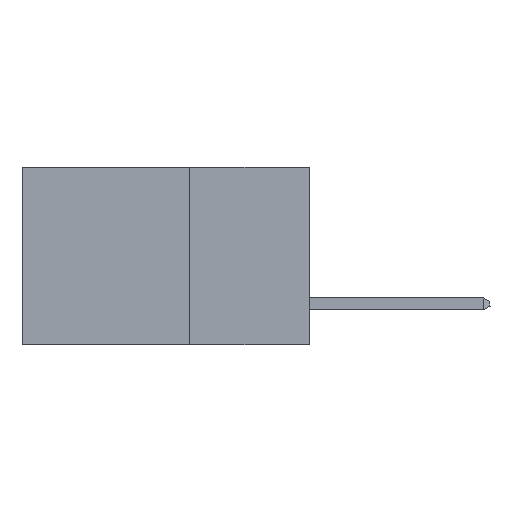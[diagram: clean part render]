
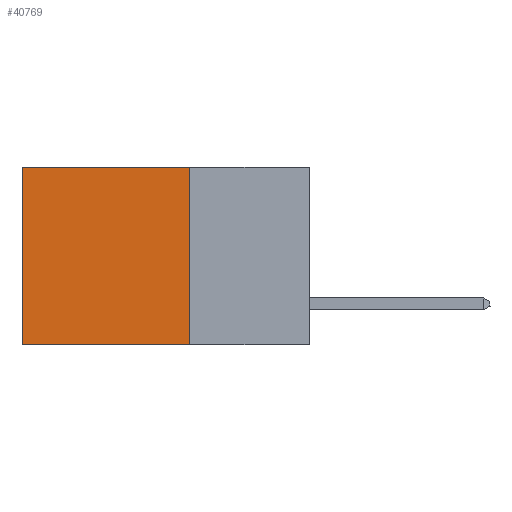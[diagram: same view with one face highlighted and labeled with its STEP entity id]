
A CAD part, left-side view. The second image highlights one B-rep face of the part: STEP entity #40769.
In plain terms, the highlighted planar face has unit normal (-1, 0, 0).
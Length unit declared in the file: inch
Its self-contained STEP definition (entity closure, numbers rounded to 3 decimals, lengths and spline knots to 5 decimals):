
#1286 = ORIENTED_EDGE ( 'NONE', *, *, #6810, .F. ) ;
#1590 = VERTEX_POINT ( 'NONE', #1863 ) ;
#1863 = CARTESIAN_POINT ( 'NONE',  ( 0.2875, 0.25, -0.37 ) ) ;
#3495 = VECTOR ( 'NONE', #34072, 39.37008 ) ;
#4183 = DIRECTION ( 'NONE',  ( 0., 1., 0. ) ) ;
#4986 = EDGE_CURVE ( 'NONE', #47253, #1590, #13332, .T. ) ;
#6810 = EDGE_CURVE ( 'NONE', #1590, #40812, #20130, .T. ) ;
#7678 = DIRECTION ( 'NONE',  ( 1., 0., 0. ) ) ;
#9888 = EDGE_LOOP ( 'NONE', ( #41208, #1286, #21151, #11912 ) ) ;
#10342 = VECTOR ( 'NONE', #39695, 39.37008 ) ;
#11912 = ORIENTED_EDGE ( 'NONE', *, *, #39698, .T. ) ;
#12501 = LINE ( 'NONE', #46012, #20705 ) ;
#13260 = FACE_OUTER_BOUND ( 'NONE', #9888, .T. ) ;
#13332 = LINE ( 'NONE', #32326, #3495 ) ;
#18733 = PLANE ( 'NONE',  #34828 ) ;
#20130 = LINE ( 'NONE', #28459, #10342 ) ;
#20638 = VERTEX_POINT ( 'NONE', #37254 ) ;
#20705 = VECTOR ( 'NONE', #45849, 39.37008 ) ;
#21151 = ORIENTED_EDGE ( 'NONE', *, *, #4986, .F. ) ;
#21906 = DIRECTION ( 'NONE',  ( 0., 0., -1. ) ) ;
#22217 = CARTESIAN_POINT ( 'NONE',  ( 0.2875, 0.25, 0. ) ) ;
#24052 = LINE ( 'NONE', #33974, #32810 ) ;
#26538 = CARTESIAN_POINT ( 'NONE',  ( 0.2875, 0.6, -0.37 ) ) ;
#28459 = CARTESIAN_POINT ( 'NONE',  ( 0.2875, 0.25, -0.37 ) ) ;
#32326 = CARTESIAN_POINT ( 'NONE',  ( 0.2875, 0.25, 0. ) ) ;
#32810 = VECTOR ( 'NONE', #4183, 39.37008 ) ;
#33974 = CARTESIAN_POINT ( 'NONE',  ( 0.2875, 0.25, 0. ) ) ;
#34072 = DIRECTION ( 'NONE',  ( 0., 0., -1. ) ) ;
#34828 = AXIS2_PLACEMENT_3D ( 'NONE', #22217, #7678, #21906 ) ;
#37254 = CARTESIAN_POINT ( 'NONE',  ( 0.2875, 0.6, 0. ) ) ;
#39695 = DIRECTION ( 'NONE',  ( 0., 1., 0. ) ) ;
#39698 = EDGE_CURVE ( 'NONE', #47253, #20638, #24052, .T. ) ;
#40360 = CARTESIAN_POINT ( 'NONE',  ( 0.2875, 0.25, 0. ) ) ;
#40769 = ADVANCED_FACE ( 'NONE', ( #13260 ), #18733, .F. ) ;
#40812 = VERTEX_POINT ( 'NONE', #26538 ) ;
#41208 = ORIENTED_EDGE ( 'NONE', *, *, #42127, .T. ) ;
#42127 = EDGE_CURVE ( 'NONE', #20638, #40812, #12501, .T. ) ;
#45849 = DIRECTION ( 'NONE',  ( 0., 0., -1. ) ) ;
#46012 = CARTESIAN_POINT ( 'NONE',  ( 0.2875, 0.6, 0. ) ) ;
#47253 = VERTEX_POINT ( 'NONE', #40360 ) ;
